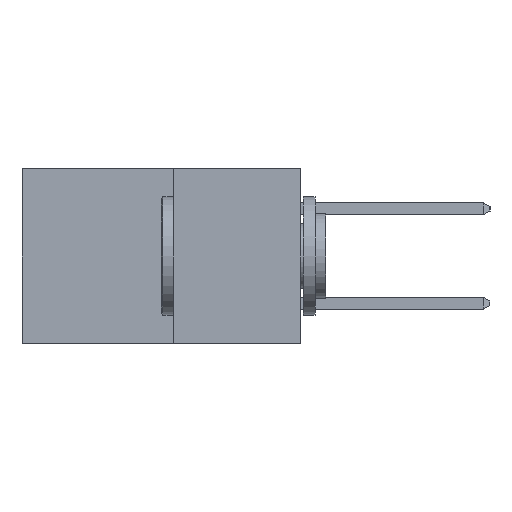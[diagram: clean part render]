
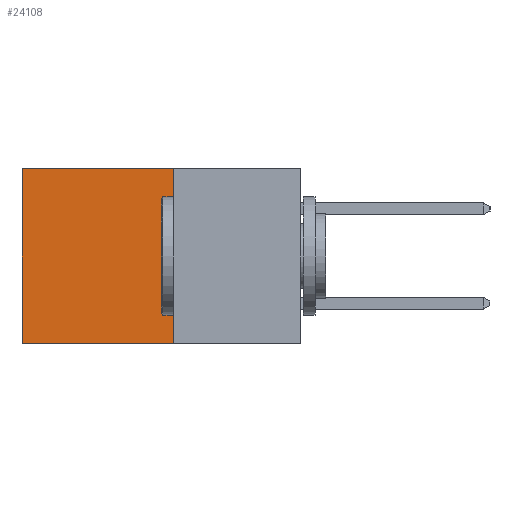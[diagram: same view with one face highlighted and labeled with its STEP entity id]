
A CAD part, left-side view. The second image highlights one B-rep face of the part: STEP entity #24108.
In plain terms, the highlighted planar face has unit normal (-1, 0, 0).
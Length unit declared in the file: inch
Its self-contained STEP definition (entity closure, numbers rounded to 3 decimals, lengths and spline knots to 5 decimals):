
#295 = VECTOR ( 'NONE', #23527, 39.37008 ) ;
#334 = LINE ( 'NONE', #1441, #24323 ) ;
#680 = EDGE_LOOP ( 'NONE', ( #8260, #1778, #14496, #19015 ) ) ;
#1441 = CARTESIAN_POINT ( 'NONE',  ( 0.277, 0.27, -0.37 ) ) ;
#1446 = CARTESIAN_POINT ( 'NONE',  ( 0.277, 0.27, 0. ) ) ;
#1498 = CARTESIAN_POINT ( 'NONE',  ( 0.277, 0.59, -0.37 ) ) ;
#1778 = ORIENTED_EDGE ( 'NONE', *, *, #5818, .F. ) ;
#2825 = VERTEX_POINT ( 'NONE', #1498 ) ;
#4638 = DIRECTION ( 'NONE',  ( 0., 1., 0. ) ) ;
#5107 = CARTESIAN_POINT ( 'NONE',  ( 0.277, 0.27, -0.37 ) ) ;
#5818 = EDGE_CURVE ( 'NONE', #18261, #2825, #334, .T. ) ;
#7720 = CARTESIAN_POINT ( 'NONE',  ( 0.277, 0.27, 0. ) ) ;
#8021 = EDGE_CURVE ( 'NONE', #15727, #2825, #15469, .T. ) ;
#8252 = VECTOR ( 'NONE', #22381, 39.37008 ) ;
#8260 = ORIENTED_EDGE ( 'NONE', *, *, #8021, .T. ) ;
#8625 = CARTESIAN_POINT ( 'NONE',  ( 0.277, 0.27, -0.37 ) ) ;
#10536 = DIRECTION ( 'NONE',  ( 0., 0., -1. ) ) ;
#10613 = VECTOR ( 'NONE', #12844, 39.37008 ) ;
#12250 = CARTESIAN_POINT ( 'NONE',  ( 0.277, 0.59, -0.37 ) ) ;
#12380 = FACE_OUTER_BOUND ( 'NONE', #680, .T. ) ;
#12844 = DIRECTION ( 'NONE',  ( 0., 1., 0. ) ) ;
#14496 = ORIENTED_EDGE ( 'NONE', *, *, #19731, .F. ) ;
#15469 = LINE ( 'NONE', #12250, #295 ) ;
#15727 = VERTEX_POINT ( 'NONE', #22118 ) ;
#16064 = AXIS2_PLACEMENT_3D ( 'NONE', #8625, #21797, #10536 ) ;
#18261 = VERTEX_POINT ( 'NONE', #5107 ) ;
#19015 = ORIENTED_EDGE ( 'NONE', *, *, #24239, .T. ) ;
#19440 = LINE ( 'NONE', #1446, #10613 ) ;
#19731 = EDGE_CURVE ( 'NONE', #24308, #18261, #23287, .T. ) ;
#21797 = DIRECTION ( 'NONE',  ( 1., 0., 0. ) ) ;
#22118 = CARTESIAN_POINT ( 'NONE',  ( 0.277, 0.59, 0. ) ) ;
#22381 = DIRECTION ( 'NONE',  ( 0., 0., -1. ) ) ;
#22606 = CARTESIAN_POINT ( 'NONE',  ( 0.277, 0.27, -0.37 ) ) ;
#23287 = LINE ( 'NONE', #22606, #8252 ) ;
#23527 = DIRECTION ( 'NONE',  ( 0., 0., -1. ) ) ;
#23617 = PLANE ( 'NONE',  #16064 ) ;
#24108 = ADVANCED_FACE ( 'NONE', ( #12380 ), #23617, .F. ) ;
#24239 = EDGE_CURVE ( 'NONE', #24308, #15727, #19440, .T. ) ;
#24308 = VERTEX_POINT ( 'NONE', #7720 ) ;
#24323 = VECTOR ( 'NONE', #4638, 39.37008 ) ;
